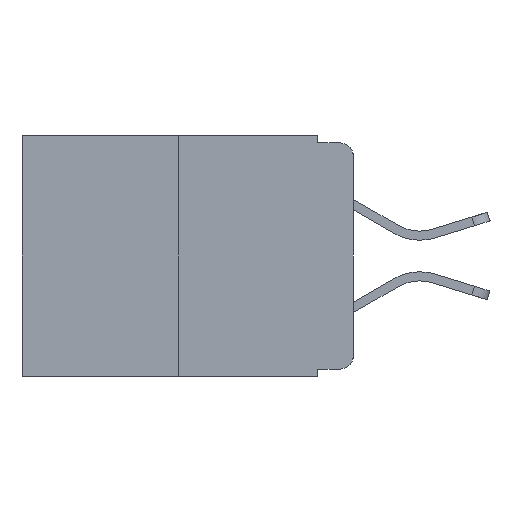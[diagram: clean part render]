
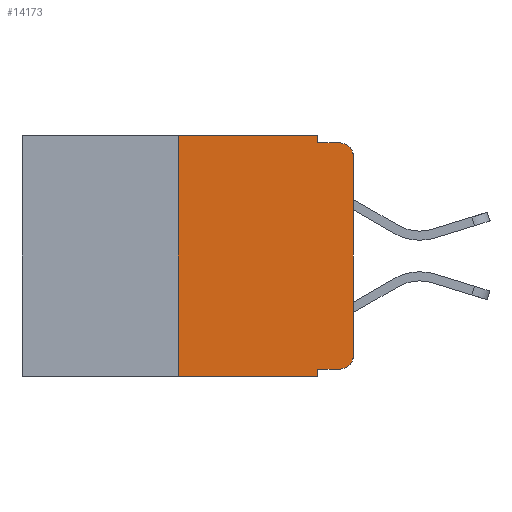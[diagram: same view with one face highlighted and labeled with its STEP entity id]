
A CAD part, left-side view. The second image highlights one B-rep face of the part: STEP entity #14173.
In plain terms, the highlighted planar face has unit normal (-1, 0, 0).
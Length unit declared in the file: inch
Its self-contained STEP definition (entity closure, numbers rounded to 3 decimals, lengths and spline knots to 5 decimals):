
#510 = CARTESIAN_POINT ( 'NONE',  ( 0., 0.02, -0.01 ) ) ;
#1116 = EDGE_CURVE ( 'NONE', #13582, #2305, #15328, .T. ) ;
#1145 = CARTESIAN_POINT ( 'NONE',  ( 0., 0.051, -0.333 ) ) ;
#1680 = VECTOR ( 'NONE', #9071, 39.37008 ) ;
#1682 = CARTESIAN_POINT ( 'NONE',  ( 0., 0.02, -0.03 ) ) ;
#1689 = VERTEX_POINT ( 'NONE', #12022 ) ;
#2059 = EDGE_CURVE ( 'NONE', #8380, #2972, #14729, .T. ) ;
#2305 = VERTEX_POINT ( 'NONE', #15657 ) ;
#2363 = CARTESIAN_POINT ( 'NONE',  ( 0., 0.051, 0. ) ) ;
#2410 = EDGE_CURVE ( 'NONE', #11936, #12959, #9836, .T. ) ;
#2618 = CARTESIAN_POINT ( 'NONE',  ( 0., 0., -0.03 ) ) ;
#2803 = CARTESIAN_POINT ( 'NONE',  ( 0., 0., -0.313 ) ) ;
#2871 = DIRECTION ( 'NONE',  ( -1., 0., 0. ) ) ;
#2899 = VERTEX_POINT ( 'NONE', #10144 ) ;
#2935 = ORIENTED_EDGE ( 'NONE', *, *, #12387, .F. ) ;
#2972 = VERTEX_POINT ( 'NONE', #510 ) ;
#3889 = EDGE_CURVE ( 'NONE', #2305, #2972, #15588, .T. ) ;
#4177 = DIRECTION ( 'NONE',  ( 0., 0., 1. ) ) ;
#4567 = VECTOR ( 'NONE', #6992, 39.37008 ) ;
#4689 = DIRECTION ( 'NONE',  ( 1., 0., 0. ) ) ;
#4768 = LINE ( 'NONE', #7826, #1680 ) ;
#4914 = FACE_OUTER_BOUND ( 'NONE', #12783, .T. ) ;
#5359 = AXIS2_PLACEMENT_3D ( 'NONE', #14439, #4689, #13319 ) ;
#5360 = DIRECTION ( 'NONE',  ( 0., 0., -1. ) ) ;
#5488 = EDGE_CURVE ( 'NONE', #2899, #12959, #8050, .T. ) ;
#5633 = VECTOR ( 'NONE', #12295, 39.37008 ) ;
#5964 = ORIENTED_EDGE ( 'NONE', *, *, #6128, .F. ) ;
#6082 = VECTOR ( 'NONE', #4177, 39.37008 ) ;
#6128 = EDGE_CURVE ( 'NONE', #11936, #1689, #12226, .T. ) ;
#6665 = CIRCLE ( 'NONE', #15269, 0.02 ) ;
#6950 = AXIS2_PLACEMENT_3D ( 'NONE', #1682, #2871, #5360 ) ;
#6992 = DIRECTION ( 'NONE',  ( 0., -1., 0. ) ) ;
#7051 = DIRECTION ( 'NONE',  ( -1., 0., 0. ) ) ;
#7344 = ORIENTED_EDGE ( 'NONE', *, *, #15768, .T. ) ;
#7804 = VECTOR ( 'NONE', #8069, 39.37008 ) ;
#7826 = CARTESIAN_POINT ( 'NONE',  ( 0., 0.473, 0. ) ) ;
#8050 = LINE ( 'NONE', #11446, #14460 ) ;
#8069 = DIRECTION ( 'NONE',  ( 0., 0., 1. ) ) ;
#8380 = VERTEX_POINT ( 'NONE', #2618 ) ;
#8390 = DIRECTION ( 'NONE',  ( 0., 0., -1. ) ) ;
#8421 = CARTESIAN_POINT ( 'NONE',  ( 0., 0.25, -0.343 ) ) ;
#8450 = VERTEX_POINT ( 'NONE', #2803 ) ;
#8853 = DIRECTION ( 'NONE',  ( 0., -1., 0. ) ) ;
#8862 = VERTEX_POINT ( 'NONE', #12380 ) ;
#8897 = ORIENTED_EDGE ( 'NONE', *, *, #1116, .F. ) ;
#9071 = DIRECTION ( 'NONE',  ( 0., -1., 0. ) ) ;
#9302 = CARTESIAN_POINT ( 'NONE',  ( 0., 0., 0. ) ) ;
#9434 = ORIENTED_EDGE ( 'NONE', *, *, #15648, .T. ) ;
#9447 = VECTOR ( 'NONE', #8853, 39.37008 ) ;
#9638 = ORIENTED_EDGE ( 'NONE', *, *, #5488, .F. ) ;
#9660 = DIRECTION ( 'NONE',  ( 0., -1., 0. ) ) ;
#9665 = PLANE ( 'NONE',  #5359 ) ;
#9674 = CARTESIAN_POINT ( 'NONE',  ( 0., 0.051, 0. ) ) ;
#9836 = LINE ( 'NONE', #12934, #9447 ) ;
#9933 = CARTESIAN_POINT ( 'NONE',  ( 0., 0.051, -0.01 ) ) ;
#10144 = CARTESIAN_POINT ( 'NONE',  ( 0., 0.051, -0.333 ) ) ;
#10406 = CARTESIAN_POINT ( 'NONE',  ( 0., 0.25, 0. ) ) ;
#11446 = CARTESIAN_POINT ( 'NONE',  ( 0., 0.051, 0. ) ) ;
#11564 = LINE ( 'NONE', #1145, #4567 ) ;
#11731 = ORIENTED_EDGE ( 'NONE', *, *, #2410, .T. ) ;
#11775 = EDGE_CURVE ( 'NONE', #2899, #8862, #11564, .T. ) ;
#11936 = VERTEX_POINT ( 'NONE', #8421 ) ;
#12022 = CARTESIAN_POINT ( 'NONE',  ( 0., 0.25, 0. ) ) ;
#12226 = LINE ( 'NONE', #10406, #6082 ) ;
#12295 = DIRECTION ( 'NONE',  ( 0., 0., -1. ) ) ;
#12380 = CARTESIAN_POINT ( 'NONE',  ( 0., 0.02, -0.333 ) ) ;
#12387 = EDGE_CURVE ( 'NONE', #1689, #13582, #4768, .T. ) ;
#12494 = ORIENTED_EDGE ( 'NONE', *, *, #11775, .T. ) ;
#12615 = CARTESIAN_POINT ( 'NONE',  ( 0., 0.051, -0.343 ) ) ;
#12783 = EDGE_LOOP ( 'NONE', ( #9434, #14325, #13219, #8897, #2935, #5964, #11731, #9638, #12494, #7344 ) ) ;
#12934 = CARTESIAN_POINT ( 'NONE',  ( 0., 0.473, -0.343 ) ) ;
#12959 = VERTEX_POINT ( 'NONE', #12615 ) ;
#13219 = ORIENTED_EDGE ( 'NONE', *, *, #3889, .F. ) ;
#13319 = DIRECTION ( 'NONE',  ( 0., 0., -1. ) ) ;
#13582 = VERTEX_POINT ( 'NONE', #2363 ) ;
#13865 = LINE ( 'NONE', #9302, #7804 ) ;
#14173 = ADVANCED_FACE ( 'NONE', ( #4914 ), #9665, .F. ) ;
#14288 = CARTESIAN_POINT ( 'NONE',  ( 0., 0.02, -0.313 ) ) ;
#14325 = ORIENTED_EDGE ( 'NONE', *, *, #2059, .T. ) ;
#14439 = CARTESIAN_POINT ( 'NONE',  ( 0., 0.473, 0. ) ) ;
#14460 = VECTOR ( 'NONE', #8390, 39.37008 ) ;
#14729 = CIRCLE ( 'NONE', #6950, 0.02 ) ;
#15247 = VECTOR ( 'NONE', #9660, 39.37008 ) ;
#15269 = AXIS2_PLACEMENT_3D ( 'NONE', #14288, #7051, #15480 ) ;
#15328 = LINE ( 'NONE', #9674, #5633 ) ;
#15480 = DIRECTION ( 'NONE',  ( 0., 0., -1. ) ) ;
#15588 = LINE ( 'NONE', #9933, #15247 ) ;
#15648 = EDGE_CURVE ( 'NONE', #8450, #8380, #13865, .T. ) ;
#15657 = CARTESIAN_POINT ( 'NONE',  ( 0., 0.051, -0.01 ) ) ;
#15768 = EDGE_CURVE ( 'NONE', #8862, #8450, #6665, .T. ) ;
